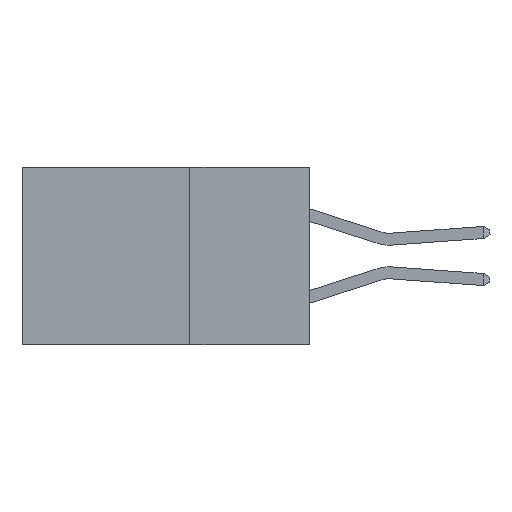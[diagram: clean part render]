
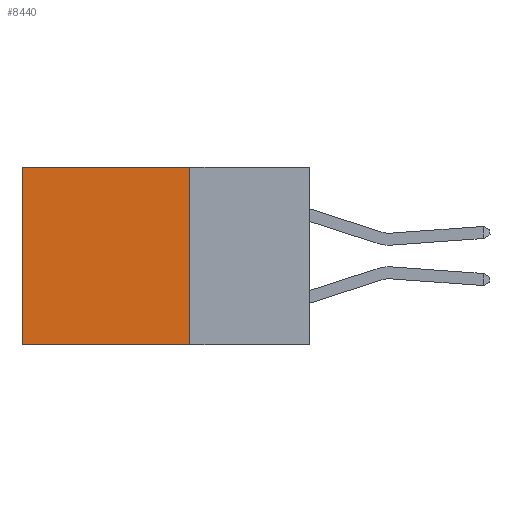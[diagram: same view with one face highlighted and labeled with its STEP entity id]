
A CAD part, left-side view. The second image highlights one B-rep face of the part: STEP entity #8440.
In plain terms, the highlighted planar face has unit normal (-1, 0, 0).
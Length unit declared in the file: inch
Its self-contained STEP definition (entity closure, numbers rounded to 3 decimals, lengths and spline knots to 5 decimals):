
#220 = DIRECTION ( 'NONE',  ( 0., 0., -1. ) ) ;
#483 = EDGE_LOOP ( 'NONE', ( #8905, #12044, #4923, #17543 ) ) ;
#604 = LINE ( 'NONE', #5249, #14737 ) ;
#630 = CARTESIAN_POINT ( 'NONE',  ( 0.298, 0.25, 0. ) ) ;
#1281 = LINE ( 'NONE', #5642, #14961 ) ;
#1398 = CARTESIAN_POINT ( 'NONE',  ( 0.298, 0.6, -0.37 ) ) ;
#2034 = PLANE ( 'NONE',  #13891 ) ;
#2608 = VERTEX_POINT ( 'NONE', #9225 ) ;
#2936 = CARTESIAN_POINT ( 'NONE',  ( 0.298, 0.6, 0. ) ) ;
#3132 = LINE ( 'NONE', #2936, #16806 ) ;
#3394 = DIRECTION ( 'NONE',  ( 0., 0., -1. ) ) ;
#4923 = ORIENTED_EDGE ( 'NONE', *, *, #6731, .F. ) ;
#5249 = CARTESIAN_POINT ( 'NONE',  ( 0.298, 0.25, 0. ) ) ;
#5642 = CARTESIAN_POINT ( 'NONE',  ( 0.298, 0.25, 0. ) ) ;
#6731 = EDGE_CURVE ( 'NONE', #7279, #2608, #604, .T. ) ;
#7279 = VERTEX_POINT ( 'NONE', #15843 ) ;
#7864 = DIRECTION ( 'NONE',  ( 0., 1., 0. ) ) ;
#8146 = CARTESIAN_POINT ( 'NONE',  ( 0.298, 0.6, 0. ) ) ;
#8440 = ADVANCED_FACE ( 'NONE', ( #11871 ), #2034, .F. ) ;
#8905 = ORIENTED_EDGE ( 'NONE', *, *, #16440, .T. ) ;
#9138 = VERTEX_POINT ( 'NONE', #1398 ) ;
#9225 = CARTESIAN_POINT ( 'NONE',  ( 0.298, 0.25, -0.37 ) ) ;
#11554 = DIRECTION ( 'NONE',  ( 1., 0., 0. ) ) ;
#11871 = FACE_OUTER_BOUND ( 'NONE', #483, .T. ) ;
#12044 = ORIENTED_EDGE ( 'NONE', *, *, #16138, .F. ) ;
#13891 = AXIS2_PLACEMENT_3D ( 'NONE', #630, #11554, #3394 ) ;
#13986 = EDGE_CURVE ( 'NONE', #7279, #14549, #1281, .T. ) ;
#14549 = VERTEX_POINT ( 'NONE', #8146 ) ;
#14737 = VECTOR ( 'NONE', #17534, 39.37008 ) ;
#14961 = VECTOR ( 'NONE', #15190, 39.37008 ) ;
#15123 = LINE ( 'NONE', #16073, #15966 ) ;
#15190 = DIRECTION ( 'NONE',  ( 0., 1., 0. ) ) ;
#15843 = CARTESIAN_POINT ( 'NONE',  ( 0.298, 0.25, 0. ) ) ;
#15966 = VECTOR ( 'NONE', #7864, 39.37008 ) ;
#16073 = CARTESIAN_POINT ( 'NONE',  ( 0.298, 0.25, -0.37 ) ) ;
#16138 = EDGE_CURVE ( 'NONE', #2608, #9138, #15123, .T. ) ;
#16440 = EDGE_CURVE ( 'NONE', #14549, #9138, #3132, .T. ) ;
#16806 = VECTOR ( 'NONE', #220, 39.37008 ) ;
#17534 = DIRECTION ( 'NONE',  ( 0., 0., -1. ) ) ;
#17543 = ORIENTED_EDGE ( 'NONE', *, *, #13986, .T. ) ;
